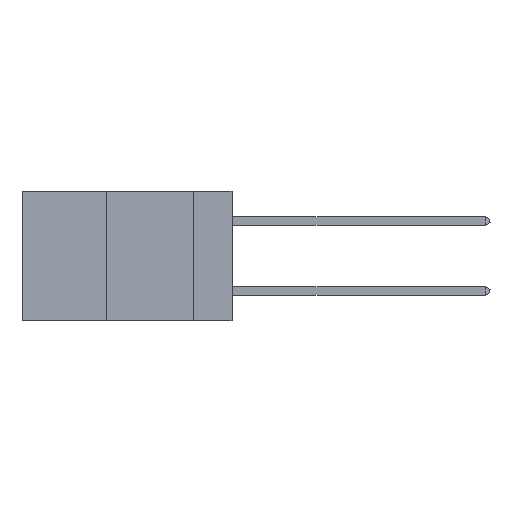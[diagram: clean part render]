
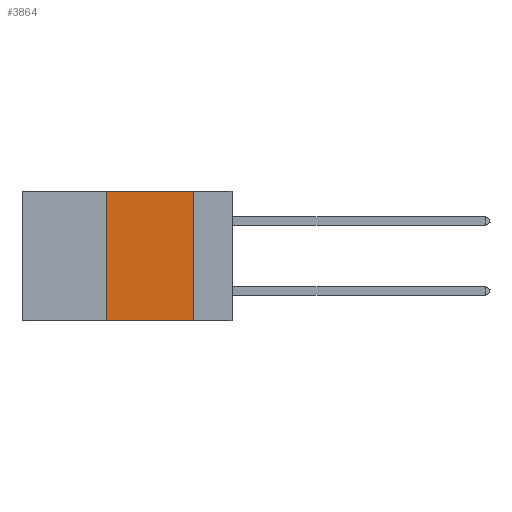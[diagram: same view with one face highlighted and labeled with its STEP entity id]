
A CAD part, left-side view. The second image highlights one B-rep face of the part: STEP entity #3864.
In plain terms, the highlighted planar face has unit normal (-1, 0, 0).
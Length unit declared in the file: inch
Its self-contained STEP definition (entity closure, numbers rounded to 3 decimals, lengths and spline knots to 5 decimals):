
#58 = VERTEX_POINT ( 'NONE', #25975 ) ;
#1048 = AXIS2_PLACEMENT_3D ( 'NONE', #5630, #29264, #38101 ) ;
#3243 = CARTESIAN_POINT ( 'NONE',  ( 0., 0.36, 0. ) ) ;
#3434 = DIRECTION ( 'NONE',  ( 0., 0., 1. ) ) ;
#3864 = ADVANCED_FACE ( 'NONE', ( #8996 ), #20597, .F. ) ;
#3898 = EDGE_CURVE ( 'NONE', #30278, #19609, #24970, .T. ) ;
#4284 = LINE ( 'NONE', #28339, #34877 ) ;
#5630 = CARTESIAN_POINT ( 'NONE',  ( 0., 0.6, 0. ) ) ;
#7474 = CARTESIAN_POINT ( 'NONE',  ( 0., 0.6, 0. ) ) ;
#8996 = FACE_OUTER_BOUND ( 'NONE', #29199, .T. ) ;
#9042 = VECTOR ( 'NONE', #25912, 39.37008 ) ;
#9787 = CARTESIAN_POINT ( 'NONE',  ( 0., 0.36, 0. ) ) ;
#13412 = DIRECTION ( 'NONE',  ( 0., -1., 0. ) ) ;
#13777 = LINE ( 'NONE', #37887, #9042 ) ;
#14380 = ORIENTED_EDGE ( 'NONE', *, *, #16094, .T. ) ;
#16077 = VECTOR ( 'NONE', #13412, 39.37008 ) ;
#16094 = EDGE_CURVE ( 'NONE', #36990, #58, #4284, .T. ) ;
#16286 = DIRECTION ( 'NONE',  ( 0., -1., 0. ) ) ;
#19100 = ORIENTED_EDGE ( 'NONE', *, *, #30555, .F. ) ;
#19609 = VERTEX_POINT ( 'NONE', #31139 ) ;
#20597 = PLANE ( 'NONE',  #1048 ) ;
#22120 = EDGE_CURVE ( 'NONE', #36990, #30278, #31902, .T. ) ;
#24970 = LINE ( 'NONE', #7474, #16077 ) ;
#25912 = DIRECTION ( 'NONE',  ( 0., 0., -1. ) ) ;
#25975 = CARTESIAN_POINT ( 'NONE',  ( 0., 0.11, -0.37 ) ) ;
#28339 = CARTESIAN_POINT ( 'NONE',  ( 0., 0.6, -0.37 ) ) ;
#29199 = EDGE_LOOP ( 'NONE', ( #19100, #37108, #36456, #14380 ) ) ;
#29264 = DIRECTION ( 'NONE',  ( 1., 0., 0. ) ) ;
#30278 = VERTEX_POINT ( 'NONE', #3243 ) ;
#30496 = CARTESIAN_POINT ( 'NONE',  ( 0., 0.36, -0.37 ) ) ;
#30555 = EDGE_CURVE ( 'NONE', #19609, #58, #13777, .T. ) ;
#31139 = CARTESIAN_POINT ( 'NONE',  ( 0., 0.11, 0. ) ) ;
#31427 = VECTOR ( 'NONE', #3434, 39.37008 ) ;
#31902 = LINE ( 'NONE', #9787, #31427 ) ;
#34877 = VECTOR ( 'NONE', #16286, 39.37008 ) ;
#36456 = ORIENTED_EDGE ( 'NONE', *, *, #22120, .F. ) ;
#36990 = VERTEX_POINT ( 'NONE', #30496 ) ;
#37108 = ORIENTED_EDGE ( 'NONE', *, *, #3898, .F. ) ;
#37887 = CARTESIAN_POINT ( 'NONE',  ( 0., 0.11, 0. ) ) ;
#38101 = DIRECTION ( 'NONE',  ( 0., 0., -1. ) ) ;
